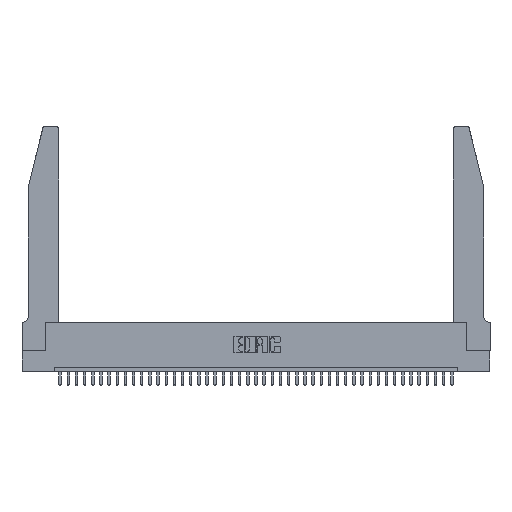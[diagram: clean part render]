
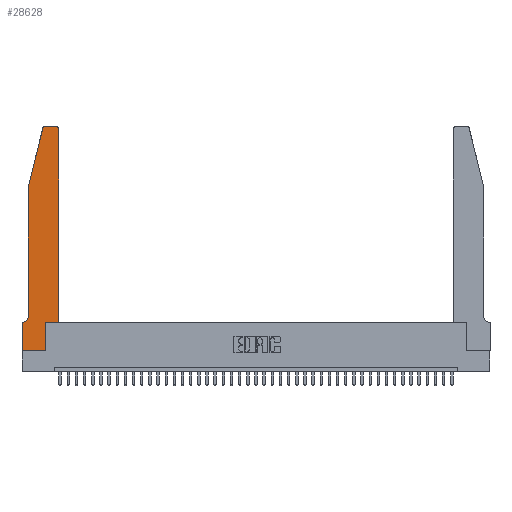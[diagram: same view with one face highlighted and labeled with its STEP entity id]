
A CAD part, top view. The second image highlights one B-rep face of the part: STEP entity #28628.
In plain terms, the highlighted planar face has unit normal (0, 0, 1).
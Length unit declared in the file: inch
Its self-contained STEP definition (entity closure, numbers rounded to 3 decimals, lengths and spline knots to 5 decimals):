
#182 = LINE ( 'NONE', #39880, #33745 ) ;
#544 = EDGE_CURVE ( 'NONE', #27667, #21117, #12487, .T. ) ;
#634 = VERTEX_POINT ( 'NONE', #23116 ) ;
#1089 = CARTESIAN_POINT ( 'NONE',  ( 0.25487, 2.72718, 0.37 ) ) ;
#1156 = CARTESIAN_POINT ( 'NONE',  ( 0.284, 2.75, 0.37 ) ) ;
#1766 = VERTEX_POINT ( 'NONE', #6282 ) ;
#2273 = EDGE_CURVE ( 'NONE', #634, #15419, #3228, .T. ) ;
#2411 = AXIS2_PLACEMENT_3D ( 'NONE', #19819, #20376, #23409 ) ;
#2489 = FACE_OUTER_BOUND ( 'NONE', #5171, .T. ) ;
#3204 = DIRECTION ( 'NONE',  ( 0., -1., 0. ) ) ;
#3228 = CIRCLE ( 'NONE', #2411, 0.07 ) ;
#3232 = VECTOR ( 'NONE', #36899, 39.37008 ) ;
#4685 = ORIENTED_EDGE ( 'NONE', *, *, #19745, .T. ) ;
#4868 = CARTESIAN_POINT ( 'NONE',  ( 0.0755, 0.35, 0.37 ) ) ;
#5171 = EDGE_LOOP ( 'NONE', ( #35971, #4685, #15989, #38673, #35243, #30793, #5527, #13707, #29383, #28356, #31583, #18101 ) ) ;
#5507 = CARTESIAN_POINT ( 'NONE',  ( 0.4505, 0.35, 0.37 ) ) ;
#5527 = ORIENTED_EDGE ( 'NONE', *, *, #14466, .T. ) ;
#6282 = CARTESIAN_POINT ( 'NONE',  ( 0.4205, 2.75, 0.37 ) ) ;
#6675 = VECTOR ( 'NONE', #3204, 39.37008 ) ;
#7099 = CARTESIAN_POINT ( 'NONE',  ( 0.0755, 2., 0.37 ) ) ;
#7132 = EDGE_CURVE ( 'NONE', #30034, #1766, #40205, .T. ) ;
#8235 = EDGE_CURVE ( 'NONE', #27577, #634, #14129, .T. ) ;
#8330 = LINE ( 'NONE', #4868, #39811 ) ;
#10246 = CARTESIAN_POINT ( 'NONE',  ( 0., 0., 0.37 ) ) ;
#10630 = DIRECTION ( 'NONE',  ( 1., 0., 0. ) ) ;
#11001 = VERTEX_POINT ( 'NONE', #17632 ) ;
#11593 = LINE ( 'NONE', #5507, #3232 ) ;
#12487 = LINE ( 'NONE', #24399, #18913 ) ;
#12603 = EDGE_CURVE ( 'NONE', #15419, #14016, #8330, .T. ) ;
#13688 = CARTESIAN_POINT ( 'NONE',  ( 0., 0., 0.37 ) ) ;
#13707 = ORIENTED_EDGE ( 'NONE', *, *, #23696, .T. ) ;
#13766 = DIRECTION ( 'NONE',  ( 0., 0., 1. ) ) ;
#14016 = VERTEX_POINT ( 'NONE', #40327 ) ;
#14102 = DIRECTION ( 'NONE',  ( -0.239, -0.971, 0. ) ) ;
#14129 = LINE ( 'NONE', #7099, #35239 ) ;
#14324 = CARTESIAN_POINT ( 'NONE',  ( 0.284, 2.72, 0.37 ) ) ;
#14466 = EDGE_CURVE ( 'NONE', #14016, #22120, #18060, .T. ) ;
#15419 = VERTEX_POINT ( 'NONE', #32205 ) ;
#15989 = ORIENTED_EDGE ( 'NONE', *, *, #36768, .T. ) ;
#17632 = CARTESIAN_POINT ( 'NONE',  ( 0.2865, 0., 0.37 ) ) ;
#17673 = DIRECTION ( 'NONE',  ( 1., 0., 0. ) ) ;
#18060 = LINE ( 'NONE', #23618, #6675 ) ;
#18101 = ORIENTED_EDGE ( 'NONE', *, *, #7132, .T. ) ;
#18913 = VECTOR ( 'NONE', #17673, 39.37008 ) ;
#19157 = CIRCLE ( 'NONE', #26619, 0.03 ) ;
#19745 = EDGE_CURVE ( 'NONE', #39527, #26549, #19157, .T. ) ;
#19819 = CARTESIAN_POINT ( 'NONE',  ( 0.0055, 0.42, 0.37 ) ) ;
#20258 = DIRECTION ( 'NONE',  ( 1., 0., 0. ) ) ;
#20376 = DIRECTION ( 'NONE',  ( 0., 0., -1. ) ) ;
#20615 = DIRECTION ( 'NONE',  ( 0., 0., 1. ) ) ;
#21117 = VERTEX_POINT ( 'NONE', #34379 ) ;
#21748 = DIRECTION ( 'NONE',  ( 0., 1., 0. ) ) ;
#22120 = VERTEX_POINT ( 'NONE', #10246 ) ;
#22913 = DIRECTION ( 'NONE',  ( 0., 0., 1. ) ) ;
#23103 = DIRECTION ( 'NONE',  ( 0., -1., 0. ) ) ;
#23116 = CARTESIAN_POINT ( 'NONE',  ( 0.0755, 0.42, 0.37 ) ) ;
#23145 = CARTESIAN_POINT ( 'NONE',  ( 0.4505, 2.72, 0.37 ) ) ;
#23409 = DIRECTION ( 'NONE',  ( -1., 0., 0. ) ) ;
#23479 = CARTESIAN_POINT ( 'NONE',  ( 0.0755, 2., 0.37 ) ) ;
#23618 = CARTESIAN_POINT ( 'NONE',  ( 0., 0., 0.37 ) ) ;
#23696 = EDGE_CURVE ( 'NONE', #22120, #11001, #37240, .T. ) ;
#24399 = CARTESIAN_POINT ( 'NONE',  ( 0.4505, 0.35, 0.37 ) ) ;
#26549 = VERTEX_POINT ( 'NONE', #1089 ) ;
#26619 = AXIS2_PLACEMENT_3D ( 'NONE', #14324, #13766, #20258 ) ;
#27577 = VERTEX_POINT ( 'NONE', #30641 ) ;
#27667 = VERTEX_POINT ( 'NONE', #28042 ) ;
#28042 = CARTESIAN_POINT ( 'NONE',  ( 0.2865, 0.35, 0.37 ) ) ;
#28125 = AXIS2_PLACEMENT_3D ( 'NONE', #36520, #20615, #36256 ) ;
#28356 = ORIENTED_EDGE ( 'NONE', *, *, #544, .T. ) ;
#28628 = ADVANCED_FACE ( 'NONE', ( #2489 ), #39665, .T. ) ;
#29383 = ORIENTED_EDGE ( 'NONE', *, *, #39934, .T. ) ;
#29596 = CARTESIAN_POINT ( 'NONE',  ( 0.4205, 2.72, 0.37 ) ) ;
#30022 = VECTOR ( 'NONE', #14102, 39.37008 ) ;
#30034 = VERTEX_POINT ( 'NONE', #23145 ) ;
#30216 = AXIS2_PLACEMENT_3D ( 'NONE', #29596, #22913, #38781 ) ;
#30493 = CARTESIAN_POINT ( 'NONE',  ( 0.2865, 0.35, 0.37 ) ) ;
#30641 = CARTESIAN_POINT ( 'NONE',  ( 0.0755, 2., 0.37 ) ) ;
#30793 = ORIENTED_EDGE ( 'NONE', *, *, #12603, .T. ) ;
#30815 = DIRECTION ( 'NONE',  ( -1., 0., 0. ) ) ;
#31583 = ORIENTED_EDGE ( 'NONE', *, *, #39147, .T. ) ;
#31680 = DIRECTION ( 'NONE',  ( -1., 0., 0. ) ) ;
#32205 = CARTESIAN_POINT ( 'NONE',  ( 0.0055, 0.35, 0.37 ) ) ;
#32629 = EDGE_CURVE ( 'NONE', #1766, #39527, #182, .T. ) ;
#32657 = LINE ( 'NONE', #30493, #38030 ) ;
#33745 = VECTOR ( 'NONE', #30815, 39.37008 ) ;
#33818 = VECTOR ( 'NONE', #10630, 39.37008 ) ;
#34379 = CARTESIAN_POINT ( 'NONE',  ( 0.4505, 0.35, 0.37 ) ) ;
#35239 = VECTOR ( 'NONE', #23103, 39.37008 ) ;
#35243 = ORIENTED_EDGE ( 'NONE', *, *, #2273, .T. ) ;
#35971 = ORIENTED_EDGE ( 'NONE', *, *, #32629, .T. ) ;
#36256 = DIRECTION ( 'NONE',  ( 1., 0., 0. ) ) ;
#36520 = CARTESIAN_POINT ( 'NONE',  ( 0., 0.35, 0.37 ) ) ;
#36768 = EDGE_CURVE ( 'NONE', #26549, #27577, #39353, .T. ) ;
#36899 = DIRECTION ( 'NONE',  ( 0., 1., 0. ) ) ;
#37240 = LINE ( 'NONE', #13688, #33818 ) ;
#38030 = VECTOR ( 'NONE', #21748, 39.37008 ) ;
#38673 = ORIENTED_EDGE ( 'NONE', *, *, #8235, .T. ) ;
#38781 = DIRECTION ( 'NONE',  ( 1., 0., 0. ) ) ;
#39147 = EDGE_CURVE ( 'NONE', #21117, #30034, #11593, .T. ) ;
#39353 = LINE ( 'NONE', #23479, #30022 ) ;
#39527 = VERTEX_POINT ( 'NONE', #1156 ) ;
#39665 = PLANE ( 'NONE',  #28125 ) ;
#39811 = VECTOR ( 'NONE', #31680, 39.37008 ) ;
#39880 = CARTESIAN_POINT ( 'NONE',  ( 0.2605, 2.75, 0.37 ) ) ;
#39934 = EDGE_CURVE ( 'NONE', #11001, #27667, #32657, .T. ) ;
#40205 = CIRCLE ( 'NONE', #30216, 0.03 ) ;
#40327 = CARTESIAN_POINT ( 'NONE',  ( 0., 0.35, 0.37 ) ) ;
